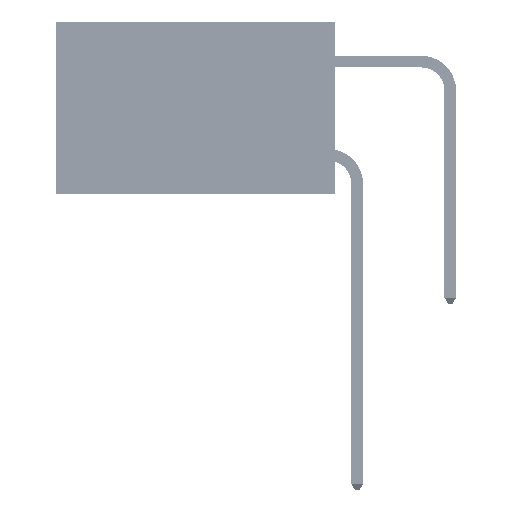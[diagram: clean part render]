
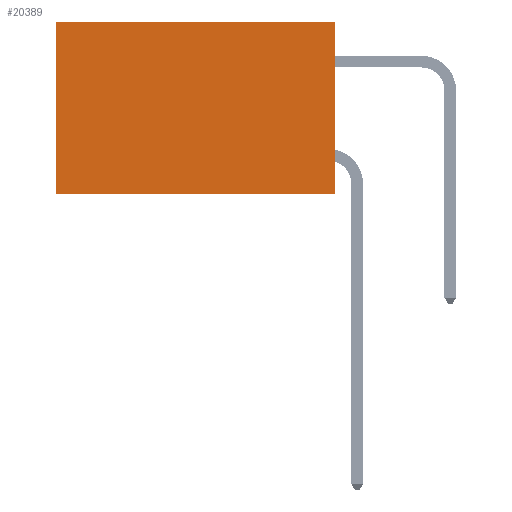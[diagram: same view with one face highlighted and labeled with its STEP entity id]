
A CAD part, left-side view. The second image highlights one B-rep face of the part: STEP entity #20389.
In plain terms, the highlighted planar face has unit normal (-1, 0, 0).
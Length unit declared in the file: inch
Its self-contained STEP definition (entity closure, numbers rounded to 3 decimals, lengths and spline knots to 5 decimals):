
#2659 = ORIENTED_EDGE ( 'NONE', *, *, #29716, .F. ) ;
#3956 = LINE ( 'NONE', #48271, #21203 ) ;
#5488 = DIRECTION ( 'NONE',  ( 0., 1., 0. ) ) ;
#5829 = DIRECTION ( 'NONE',  ( 1., 0., 0. ) ) ;
#6043 = EDGE_CURVE ( 'NONE', #38244, #45357, #35029, .T. ) ;
#9680 = CARTESIAN_POINT ( 'NONE',  ( 0.2875, 0., -0.37 ) ) ;
#10682 = VERTEX_POINT ( 'NONE', #22224 ) ;
#10758 = CARTESIAN_POINT ( 'NONE',  ( 0.2875, 0.6, -0.37 ) ) ;
#11553 = FACE_OUTER_BOUND ( 'NONE', #47182, .T. ) ;
#15568 = AXIS2_PLACEMENT_3D ( 'NONE', #24795, #5829, #16848 ) ;
#16848 = DIRECTION ( 'NONE',  ( 0., 0., -1. ) ) ;
#20224 = CARTESIAN_POINT ( 'NONE',  ( 0.2875, 0., -0.37 ) ) ;
#20302 = EDGE_CURVE ( 'NONE', #44722, #45357, #48438, .T. ) ;
#20389 = ADVANCED_FACE ( 'NONE', ( #11553 ), #47931, .F. ) ;
#21203 = VECTOR ( 'NONE', #29959, 39.37008 ) ;
#22224 = CARTESIAN_POINT ( 'NONE',  ( 0.2875, 0., 0. ) ) ;
#24795 = CARTESIAN_POINT ( 'NONE',  ( 0.2875, 0., 0. ) ) ;
#25980 = DIRECTION ( 'NONE',  ( 0., 1., 0. ) ) ;
#27499 = DIRECTION ( 'NONE',  ( 0., 0., -1. ) ) ;
#29167 = LINE ( 'NONE', #41509, #31606 ) ;
#29716 = EDGE_CURVE ( 'NONE', #10682, #38244, #3956, .T. ) ;
#29959 = DIRECTION ( 'NONE',  ( 0., 0., -1. ) ) ;
#30200 = VECTOR ( 'NONE', #5488, 39.37008 ) ;
#31606 = VECTOR ( 'NONE', #25980, 39.37008 ) ;
#32003 = CARTESIAN_POINT ( 'NONE',  ( 0.2875, 0.6, 0. ) ) ;
#34862 = ORIENTED_EDGE ( 'NONE', *, *, #20302, .T. ) ;
#35029 = LINE ( 'NONE', #9680, #30200 ) ;
#35212 = CARTESIAN_POINT ( 'NONE',  ( 0.2875, 0.6, 0. ) ) ;
#37010 = ORIENTED_EDGE ( 'NONE', *, *, #48534, .T. ) ;
#38244 = VERTEX_POINT ( 'NONE', #20224 ) ;
#41509 = CARTESIAN_POINT ( 'NONE',  ( 0.2875, 0., 0. ) ) ;
#41831 = ORIENTED_EDGE ( 'NONE', *, *, #6043, .F. ) ;
#42524 = VECTOR ( 'NONE', #27499, 39.37008 ) ;
#44722 = VERTEX_POINT ( 'NONE', #35212 ) ;
#45357 = VERTEX_POINT ( 'NONE', #10758 ) ;
#47182 = EDGE_LOOP ( 'NONE', ( #34862, #41831, #2659, #37010 ) ) ;
#47931 = PLANE ( 'NONE',  #15568 ) ;
#48271 = CARTESIAN_POINT ( 'NONE',  ( 0.2875, 0., 0. ) ) ;
#48438 = LINE ( 'NONE', #32003, #42524 ) ;
#48534 = EDGE_CURVE ( 'NONE', #10682, #44722, #29167, .T. ) ;
